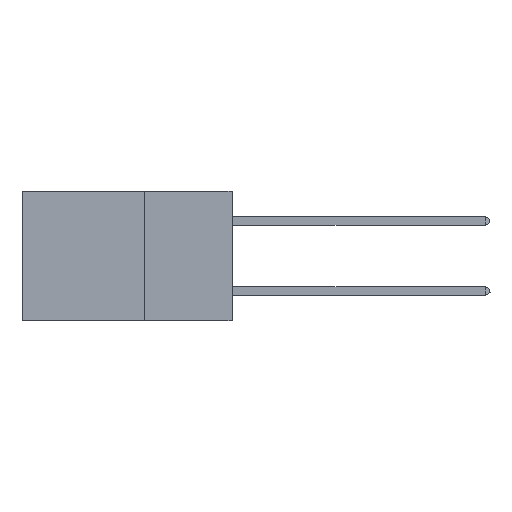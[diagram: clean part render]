
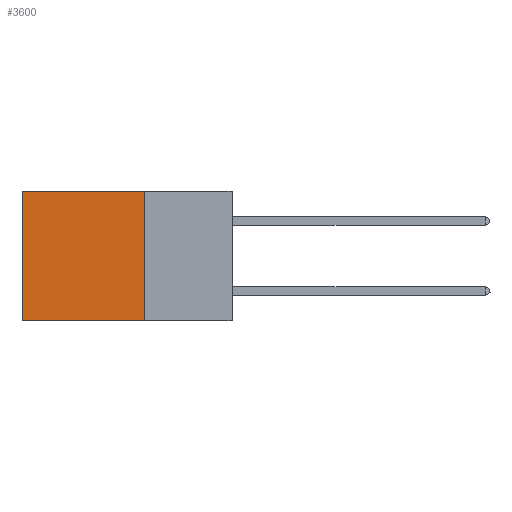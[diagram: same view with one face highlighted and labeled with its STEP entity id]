
A CAD part, left-side view. The second image highlights one B-rep face of the part: STEP entity #3600.
In plain terms, the highlighted planar face has unit normal (-1, 0, 0).
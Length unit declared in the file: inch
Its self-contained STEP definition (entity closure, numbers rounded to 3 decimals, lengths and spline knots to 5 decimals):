
#335 = LINE ( 'NONE', #12663, #12463 ) ;
#942 = LINE ( 'NONE', #12020, #13059 ) ;
#1414 = VECTOR ( 'NONE', #11854, 39.37008 ) ;
#1608 = VERTEX_POINT ( 'NONE', #6553 ) ;
#1757 = EDGE_CURVE ( 'NONE', #3730, #13935, #942, .T. ) ;
#2521 = CARTESIAN_POINT ( 'NONE',  ( 0.2875, 0.6, 0. ) ) ;
#2684 = DIRECTION ( 'NONE',  ( 0., 0., -1. ) ) ;
#3600 = ADVANCED_FACE ( 'NONE', ( #8389 ), #4900, .F. ) ;
#3724 = CARTESIAN_POINT ( 'NONE',  ( 0.2875, 0.6, -0.37 ) ) ;
#3730 = VERTEX_POINT ( 'NONE', #7023 ) ;
#4271 = EDGE_CURVE ( 'NONE', #1608, #4549, #10743, .T. ) ;
#4434 = DIRECTION ( 'NONE',  ( 0., 1., 0. ) ) ;
#4549 = VERTEX_POINT ( 'NONE', #3724 ) ;
#4900 = PLANE ( 'NONE',  #5415 ) ;
#5415 = AXIS2_PLACEMENT_3D ( 'NONE', #13120, #10790, #8631 ) ;
#6397 = DIRECTION ( 'NONE',  ( 0., 1., 0. ) ) ;
#6553 = CARTESIAN_POINT ( 'NONE',  ( 0.2875, 0.6, 0. ) ) ;
#7023 = CARTESIAN_POINT ( 'NONE',  ( 0.2875, 0.25, 0. ) ) ;
#8389 = FACE_OUTER_BOUND ( 'NONE', #12619, .T. ) ;
#8610 = CARTESIAN_POINT ( 'NONE',  ( 0.2875, 0.25, -0.37 ) ) ;
#8614 = ORIENTED_EDGE ( 'NONE', *, *, #4271, .T. ) ;
#8631 = DIRECTION ( 'NONE',  ( 0., 0., -1. ) ) ;
#9278 = VECTOR ( 'NONE', #6397, 39.37008 ) ;
#9631 = LINE ( 'NONE', #13390, #9278 ) ;
#9970 = EDGE_CURVE ( 'NONE', #3730, #1608, #335, .T. ) ;
#10743 = LINE ( 'NONE', #2521, #1414 ) ;
#10790 = DIRECTION ( 'NONE',  ( 1., 0., 0. ) ) ;
#11854 = DIRECTION ( 'NONE',  ( 0., 0., -1. ) ) ;
#11957 = EDGE_CURVE ( 'NONE', #13935, #4549, #9631, .T. ) ;
#12020 = CARTESIAN_POINT ( 'NONE',  ( 0.2875, 0.25, 0. ) ) ;
#12463 = VECTOR ( 'NONE', #4434, 39.37008 ) ;
#12619 = EDGE_LOOP ( 'NONE', ( #8614, #14523, #13989, #12811 ) ) ;
#12663 = CARTESIAN_POINT ( 'NONE',  ( 0.2875, 0.25, 0. ) ) ;
#12811 = ORIENTED_EDGE ( 'NONE', *, *, #9970, .T. ) ;
#13059 = VECTOR ( 'NONE', #2684, 39.37008 ) ;
#13120 = CARTESIAN_POINT ( 'NONE',  ( 0.2875, 0.25, 0. ) ) ;
#13390 = CARTESIAN_POINT ( 'NONE',  ( 0.2875, 0.25, -0.37 ) ) ;
#13935 = VERTEX_POINT ( 'NONE', #8610 ) ;
#13989 = ORIENTED_EDGE ( 'NONE', *, *, #1757, .F. ) ;
#14523 = ORIENTED_EDGE ( 'NONE', *, *, #11957, .F. ) ;
